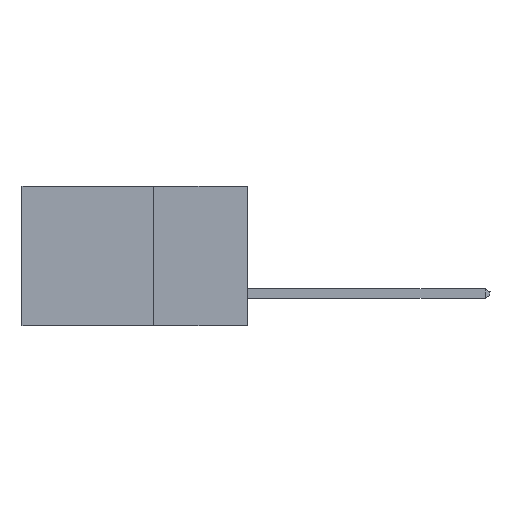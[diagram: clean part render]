
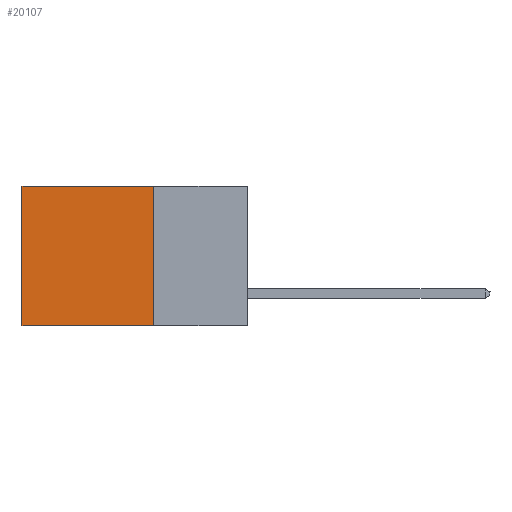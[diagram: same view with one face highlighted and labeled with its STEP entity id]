
A CAD part, left-side view. The second image highlights one B-rep face of the part: STEP entity #20107.
In plain terms, the highlighted planar face has unit normal (-1, 0, 0).
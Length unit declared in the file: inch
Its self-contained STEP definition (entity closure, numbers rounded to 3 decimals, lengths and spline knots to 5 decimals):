
#1053 = DIRECTION ( 'NONE',  ( 0., 1., 0. ) ) ;
#2165 = EDGE_CURVE ( 'NONE', #14069, #15280, #20366, .T. ) ;
#2238 = DIRECTION ( 'NONE',  ( 0., 1., 0. ) ) ;
#4155 = EDGE_CURVE ( 'NONE', #7842, #7486, #12479, .T. ) ;
#4204 = CARTESIAN_POINT ( 'NONE',  ( 0.2615, 0.25, -0.37 ) ) ;
#4941 = DIRECTION ( 'NONE',  ( 1., 0., 0. ) ) ;
#6575 = VECTOR ( 'NONE', #2238, 39.37008 ) ;
#6770 = LINE ( 'NONE', #12116, #7590 ) ;
#7486 = VERTEX_POINT ( 'NONE', #15420 ) ;
#7590 = VECTOR ( 'NONE', #10300, 39.37008 ) ;
#7633 = DIRECTION ( 'NONE',  ( 0., 0., -1. ) ) ;
#7842 = VERTEX_POINT ( 'NONE', #21154 ) ;
#8936 = EDGE_LOOP ( 'NONE', ( #22979, #19132, #20618, #10747 ) ) ;
#9464 = CARTESIAN_POINT ( 'NONE',  ( 0.2615, 0.6, 0. ) ) ;
#10026 = EDGE_CURVE ( 'NONE', #14069, #7842, #20741, .T. ) ;
#10300 = DIRECTION ( 'NONE',  ( 0., 0., -1. ) ) ;
#10747 = ORIENTED_EDGE ( 'NONE', *, *, #2165, .T. ) ;
#11732 = VECTOR ( 'NONE', #1053, 39.37008 ) ;
#12116 = CARTESIAN_POINT ( 'NONE',  ( 0.2615, 0.6, -0.37 ) ) ;
#12479 = LINE ( 'NONE', #19882, #11732 ) ;
#14069 = VERTEX_POINT ( 'NONE', #19003 ) ;
#14180 = FACE_OUTER_BOUND ( 'NONE', #8936, .T. ) ;
#15280 = VERTEX_POINT ( 'NONE', #9464 ) ;
#15420 = CARTESIAN_POINT ( 'NONE',  ( 0.2615, 0.6, -0.37 ) ) ;
#16071 = EDGE_CURVE ( 'NONE', #15280, #7486, #6770, .T. ) ;
#16136 = DIRECTION ( 'NONE',  ( 0., 0., -1. ) ) ;
#16643 = AXIS2_PLACEMENT_3D ( 'NONE', #17947, #4941, #16136 ) ;
#17947 = CARTESIAN_POINT ( 'NONE',  ( 0.2615, 0.25, -0.37 ) ) ;
#19003 = CARTESIAN_POINT ( 'NONE',  ( 0.2615, 0.25, 0. ) ) ;
#19047 = VECTOR ( 'NONE', #7633, 39.37008 ) ;
#19132 = ORIENTED_EDGE ( 'NONE', *, *, #4155, .F. ) ;
#19530 = PLANE ( 'NONE',  #16643 ) ;
#19882 = CARTESIAN_POINT ( 'NONE',  ( 0.2615, 0.25, -0.37 ) ) ;
#20107 = ADVANCED_FACE ( 'NONE', ( #14180 ), #19530, .F. ) ;
#20366 = LINE ( 'NONE', #20724, #6575 ) ;
#20618 = ORIENTED_EDGE ( 'NONE', *, *, #10026, .F. ) ;
#20724 = CARTESIAN_POINT ( 'NONE',  ( 0.2615, 0.25, 0. ) ) ;
#20741 = LINE ( 'NONE', #4204, #19047 ) ;
#21154 = CARTESIAN_POINT ( 'NONE',  ( 0.2615, 0.25, -0.37 ) ) ;
#22979 = ORIENTED_EDGE ( 'NONE', *, *, #16071, .T. ) ;
